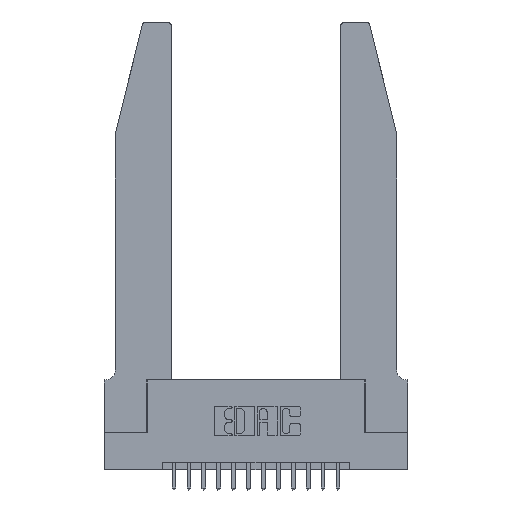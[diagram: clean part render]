
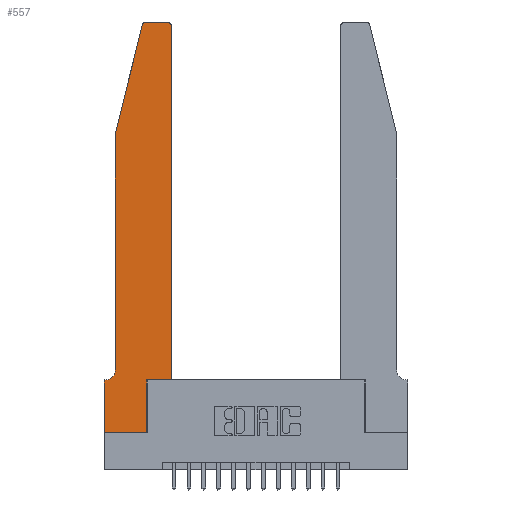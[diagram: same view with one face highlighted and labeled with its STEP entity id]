
A CAD part, top view. The second image highlights one B-rep face of the part: STEP entity #557.
In plain terms, the highlighted planar face has unit normal (0, 0, 1).
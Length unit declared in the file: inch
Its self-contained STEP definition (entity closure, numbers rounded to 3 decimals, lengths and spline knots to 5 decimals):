
#36 = DIRECTION ( 'NONE',  ( 0., -1., 0. ) ) ;
#411 = VECTOR ( 'NONE', #14845, 39.37008 ) ;
#557 = ADVANCED_FACE ( 'NONE', ( #15635 ), #15275, .T. ) ;
#575 = LINE ( 'NONE', #2541, #4074 ) ;
#664 = VECTOR ( 'NONE', #824, 39.37008 ) ;
#824 = DIRECTION ( 'NONE',  ( 1., 0., 0. ) ) ;
#966 = DIRECTION ( 'NONE',  ( -1., 0., 0. ) ) ;
#975 = EDGE_CURVE ( 'NONE', #13331, #9822, #14095, .T. ) ;
#1048 = VECTOR ( 'NONE', #36, 39.37008 ) ;
#1055 = LINE ( 'NONE', #8282, #17569 ) ;
#1076 = CARTESIAN_POINT ( 'NONE',  ( 0.0755, 0.42, 0.37 ) ) ;
#1112 = VERTEX_POINT ( 'NONE', #3839 ) ;
#1250 = VERTEX_POINT ( 'NONE', #1076 ) ;
#1989 = EDGE_CURVE ( 'NONE', #6636, #3175, #17604, .T. ) ;
#2184 = DIRECTION ( 'NONE',  ( 1., 0., 0. ) ) ;
#2211 = CARTESIAN_POINT ( 'NONE',  ( 0.25487, 2.72718, 0.37 ) ) ;
#2215 = EDGE_CURVE ( 'NONE', #9723, #1250, #3704, .T. ) ;
#2444 = VERTEX_POINT ( 'NONE', #2211 ) ;
#2541 = CARTESIAN_POINT ( 'NONE',  ( 0.0755, 0.35, 0.37 ) ) ;
#2556 = CARTESIAN_POINT ( 'NONE',  ( 0.284, 2.72, 0.37 ) ) ;
#2597 = LINE ( 'NONE', #2694, #15175 ) ;
#2694 = CARTESIAN_POINT ( 'NONE',  ( 0.2605, 2.75, 0.37 ) ) ;
#2780 = DIRECTION ( 'NONE',  ( 0., 1., 0. ) ) ;
#3071 = CARTESIAN_POINT ( 'NONE',  ( 0.0755, 2., 0.37 ) ) ;
#3175 = VERTEX_POINT ( 'NONE', #7519 ) ;
#3492 = CARTESIAN_POINT ( 'NONE',  ( 0., 0., 0.37 ) ) ;
#3529 = CIRCLE ( 'NONE', #9444, 0.03 ) ;
#3644 = CARTESIAN_POINT ( 'NONE',  ( 0.284, 2.75, 0.37 ) ) ;
#3704 = LINE ( 'NONE', #3071, #9226 ) ;
#3752 = CARTESIAN_POINT ( 'NONE',  ( 0.4505, 0.35, 0.37 ) ) ;
#3839 = CARTESIAN_POINT ( 'NONE',  ( 0.4505, 0.35, 0.37 ) ) ;
#4074 = VECTOR ( 'NONE', #966, 39.37008 ) ;
#4222 = DIRECTION ( 'NONE',  ( 0., 0., -1. ) ) ;
#4533 = VERTEX_POINT ( 'NONE', #3644 ) ;
#4544 = LINE ( 'NONE', #6954, #1048 ) ;
#5279 = EDGE_CURVE ( 'NONE', #3175, #9326, #8465, .T. ) ;
#5563 = DIRECTION ( 'NONE',  ( -1., 0., 0. ) ) ;
#6003 = ORIENTED_EDGE ( 'NONE', *, *, #9419, .T. ) ;
#6240 = CARTESIAN_POINT ( 'NONE',  ( 0.2865, 0.35, 0.37 ) ) ;
#6354 = DIRECTION ( 'NONE',  ( 0., 0., 1. ) ) ;
#6636 = VERTEX_POINT ( 'NONE', #12521 ) ;
#6718 = EDGE_CURVE ( 'NONE', #1250, #16781, #13736, .T. ) ;
#6805 = DIRECTION ( 'NONE',  ( 1., 0., 0. ) ) ;
#6954 = CARTESIAN_POINT ( 'NONE',  ( 0., 0., 0.37 ) ) ;
#7519 = CARTESIAN_POINT ( 'NONE',  ( 0.2865, 0., 0.37 ) ) ;
#7556 = AXIS2_PLACEMENT_3D ( 'NONE', #14996, #6354, #2184 ) ;
#8282 = CARTESIAN_POINT ( 'NONE',  ( 0.4505, 0.35, 0.37 ) ) ;
#8322 = VECTOR ( 'NONE', #15209, 39.37008 ) ;
#8394 = DIRECTION ( 'NONE',  ( -1., 0., 0. ) ) ;
#8465 = LINE ( 'NONE', #13238, #15355 ) ;
#9050 = ORIENTED_EDGE ( 'NONE', *, *, #15207, .T. ) ;
#9226 = VECTOR ( 'NONE', #12921, 39.37008 ) ;
#9326 = VERTEX_POINT ( 'NONE', #6240 ) ;
#9419 = EDGE_CURVE ( 'NONE', #4533, #2444, #3529, .T. ) ;
#9426 = CARTESIAN_POINT ( 'NONE',  ( 0.0055, 0.35, 0.37 ) ) ;
#9444 = AXIS2_PLACEMENT_3D ( 'NONE', #2556, #15192, #11031 ) ;
#9574 = CARTESIAN_POINT ( 'NONE',  ( 0., 0.35, 0.37 ) ) ;
#9710 = DIRECTION ( 'NONE',  ( 1., 0., 0. ) ) ;
#9723 = VERTEX_POINT ( 'NONE', #17657 ) ;
#9822 = VERTEX_POINT ( 'NONE', #10881 ) ;
#9858 = LINE ( 'NONE', #10584, #411 ) ;
#9885 = ORIENTED_EDGE ( 'NONE', *, *, #1989, .T. ) ;
#9913 = AXIS2_PLACEMENT_3D ( 'NONE', #12508, #13855, #6805 ) ;
#10584 = CARTESIAN_POINT ( 'NONE',  ( 0.0755, 2., 0.37 ) ) ;
#10881 = CARTESIAN_POINT ( 'NONE',  ( 0.4205, 2.75, 0.37 ) ) ;
#11031 = DIRECTION ( 'NONE',  ( 1., 0., 0. ) ) ;
#11790 = CARTESIAN_POINT ( 'NONE',  ( 0.4505, 2.72, 0.37 ) ) ;
#11851 = LINE ( 'NONE', #3752, #8322 ) ;
#11881 = ORIENTED_EDGE ( 'NONE', *, *, #5279, .T. ) ;
#12080 = ORIENTED_EDGE ( 'NONE', *, *, #6718, .T. ) ;
#12508 = CARTESIAN_POINT ( 'NONE',  ( 0., 0.35, 0.37 ) ) ;
#12521 = CARTESIAN_POINT ( 'NONE',  ( 0., 0., 0.37 ) ) ;
#12921 = DIRECTION ( 'NONE',  ( 0., -1., 0. ) ) ;
#13057 = VERTEX_POINT ( 'NONE', #9574 ) ;
#13067 = ORIENTED_EDGE ( 'NONE', *, *, #18130, .T. ) ;
#13238 = CARTESIAN_POINT ( 'NONE',  ( 0.2865, 0.35, 0.37 ) ) ;
#13331 = VERTEX_POINT ( 'NONE', #11790 ) ;
#13524 = AXIS2_PLACEMENT_3D ( 'NONE', #18241, #4222, #5563 ) ;
#13736 = CIRCLE ( 'NONE', #13524, 0.07 ) ;
#13855 = DIRECTION ( 'NONE',  ( 0., 0., 1. ) ) ;
#14095 = CIRCLE ( 'NONE', #7556, 0.03 ) ;
#14516 = ORIENTED_EDGE ( 'NONE', *, *, #975, .T. ) ;
#14845 = DIRECTION ( 'NONE',  ( -0.239, -0.971, 0. ) ) ;
#14996 = CARTESIAN_POINT ( 'NONE',  ( 0.4205, 2.72, 0.37 ) ) ;
#15131 = ORIENTED_EDGE ( 'NONE', *, *, #2215, .T. ) ;
#15175 = VECTOR ( 'NONE', #8394, 39.37008 ) ;
#15192 = DIRECTION ( 'NONE',  ( 0., 0., 1. ) ) ;
#15207 = EDGE_CURVE ( 'NONE', #9326, #1112, #1055, .T. ) ;
#15209 = DIRECTION ( 'NONE',  ( 0., 1., 0. ) ) ;
#15275 = PLANE ( 'NONE',  #9913 ) ;
#15355 = VECTOR ( 'NONE', #2780, 39.37008 ) ;
#15635 = FACE_OUTER_BOUND ( 'NONE', #17509, .T. ) ;
#15906 = ORIENTED_EDGE ( 'NONE', *, *, #16410, .T. ) ;
#16410 = EDGE_CURVE ( 'NONE', #16781, #13057, #575, .T. ) ;
#16637 = ORIENTED_EDGE ( 'NONE', *, *, #16925, .T. ) ;
#16644 = EDGE_CURVE ( 'NONE', #2444, #9723, #9858, .T. ) ;
#16748 = EDGE_CURVE ( 'NONE', #1112, #13331, #11851, .T. ) ;
#16781 = VERTEX_POINT ( 'NONE', #9426 ) ;
#16925 = EDGE_CURVE ( 'NONE', #9822, #4533, #2597, .T. ) ;
#17353 = ORIENTED_EDGE ( 'NONE', *, *, #16644, .T. ) ;
#17509 = EDGE_LOOP ( 'NONE', ( #16637, #6003, #17353, #15131, #12080, #15906, #13067, #9885, #11881, #9050, #17543, #14516 ) ) ;
#17543 = ORIENTED_EDGE ( 'NONE', *, *, #16748, .T. ) ;
#17569 = VECTOR ( 'NONE', #9710, 39.37008 ) ;
#17604 = LINE ( 'NONE', #3492, #664 ) ;
#17657 = CARTESIAN_POINT ( 'NONE',  ( 0.0755, 2., 0.37 ) ) ;
#18130 = EDGE_CURVE ( 'NONE', #13057, #6636, #4544, .T. ) ;
#18241 = CARTESIAN_POINT ( 'NONE',  ( 0.0055, 0.42, 0.37 ) ) ;
